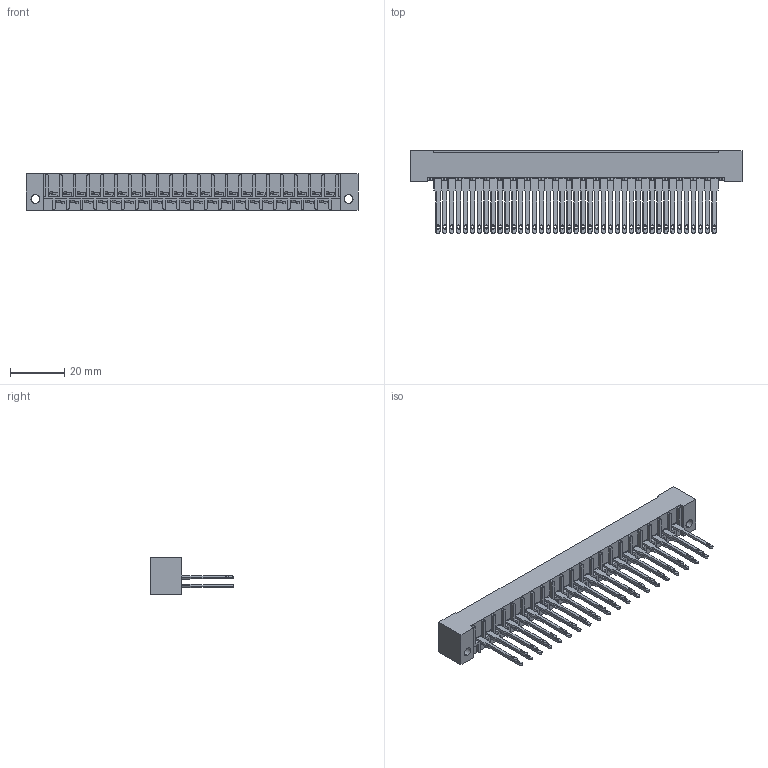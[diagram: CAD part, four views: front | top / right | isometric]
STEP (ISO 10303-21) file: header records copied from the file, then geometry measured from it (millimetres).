
FILE_DESCRIPTION (( 'STEP AP203' ), '1' );
FILE_NAME ('408-047-540-122.STEP', '2019-11-04T19:52:04', ( '' ), ( '' ), 'SwSTEP 2.0', 'SolidWorks 2016', '' );
FILE_SCHEMA (( 'CONFIG_CONTROL_DESIGN' ));
Length unit declared in the file: inch
Products named in the file (3): 408 Part_041 - 1; 408-290-001_408-290-140; 408-047-540-122
Assembly tree (42 placements, depth 2):
  408-047-540-122
    408 Part_041 - 1
    408-290-001_408-290-140  x41
Bounding box: 122.07 x 30.4 x 13.49 mm (x, y, z)
Volume: 14014.1 mm3; surface area: 19790.9 mm2
Topology: 42 solids, 42 shells, 2381 faces, 6559 edges, 4262 vertices
Faces by surface type: plane 1758, cylinder 459, bspline 164
Entity records: 27570 total; most frequent: CARTESIAN_POINT 4743, ORIENTED_EDGE 4638, DIRECTION 4153, EDGE_CURVE 2319, LINE 2121, VECTOR 2121, VERTEX_POINT 1542, AXIS2_PLACEMENT_3D 1016
